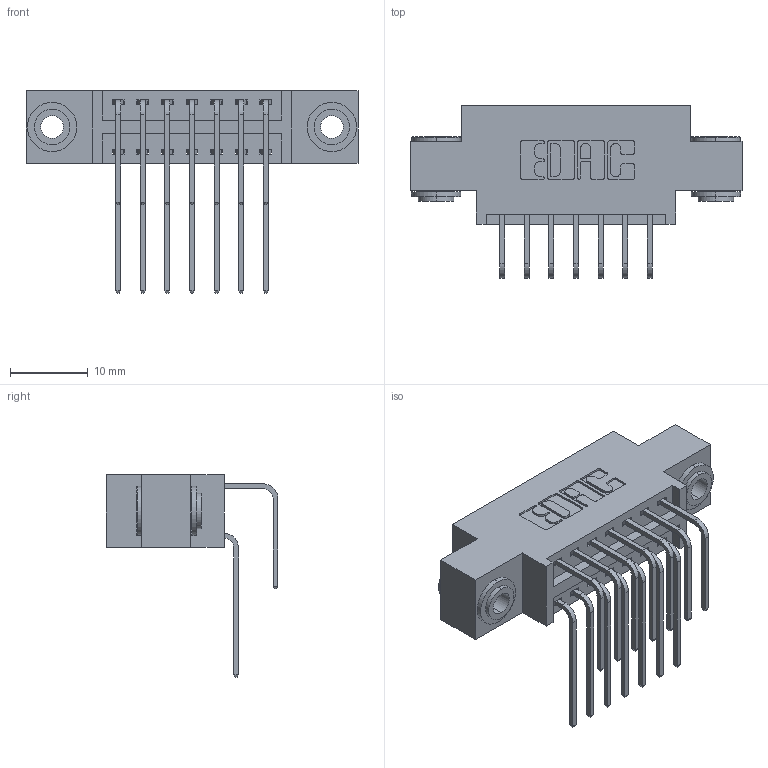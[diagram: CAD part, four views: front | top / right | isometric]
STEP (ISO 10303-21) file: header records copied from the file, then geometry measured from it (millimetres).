
FILE_DESCRIPTION (( 'STEP AP203' ), '1' );
FILE_NAME ('396-014-558-803.STEP', '2018-08-31T11:02:56', ( '' ), ( '' ), 'SwSTEP 2.0', 'SolidWorks 2016', '' );
FILE_SCHEMA (( 'CONFIG_CONTROL_DESIGN' ));
Length unit declared in the file: inch
Products named in the file (5): 345-292-001_558 Tail - 2; 345-250-002_345-250-002-102; 396-014-558-803; 346 Part_0.170 Offset - 0.156 Dia-TH; 345-292-001_558 559 Tail - 1
Assembly tree (17 placements, depth 2):
  396-014-558-803
    346 Part_0.170 Offset - 0.156 Dia-TH
    345-292-001_558 559 Tail - 1  x7
    345-292-001_558 Tail - 2  x7
    345-250-002_345-250-002-102  x2
Bounding box: 42.8 x 22.16 x 26.16 mm (x, y, z)
Volume: 3847.1 mm3; surface area: 5519.3 mm2
Topology: 17 solids, 17 shells, 920 faces, 2671 edges, 1758 vertices
Faces by surface type: plane 608, cylinder 304, cone 8
Entity records: 11846 total; most frequent: CARTESIAN_POINT 2030, ORIENTED_EDGE 1906, DIRECTION 1843, EDGE_CURVE 953, LINE 729, VECTOR 729, VERTEX_POINT 630, AXIS2_PLACEMENT_3D 557
